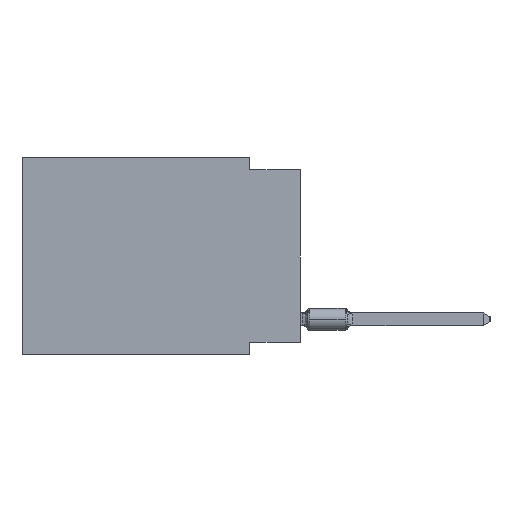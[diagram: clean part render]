
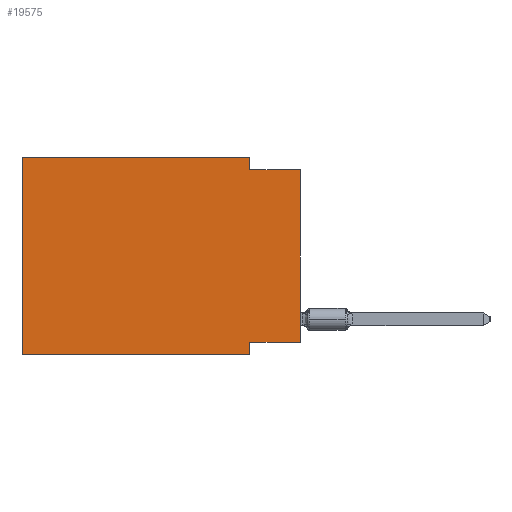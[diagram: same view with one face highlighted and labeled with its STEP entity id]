
A CAD part, left-side view. The second image highlights one B-rep face of the part: STEP entity #19575.
In plain terms, the highlighted planar face has unit normal (-1, 0, 0).
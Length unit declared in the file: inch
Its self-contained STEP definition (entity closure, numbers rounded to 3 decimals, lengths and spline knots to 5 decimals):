
#99 = CARTESIAN_POINT ( 'NONE',  ( 0., 0.1, -0.365 ) ) ;
#309 = EDGE_CURVE ( 'NONE', #10450, #14583, #4186, .T. ) ;
#503 = LINE ( 'NONE', #7809, #4864 ) ;
#529 = DIRECTION ( 'NONE',  ( 1., 0., 0. ) ) ;
#1106 = ORIENTED_EDGE ( 'NONE', *, *, #4842, .T. ) ;
#1479 = CARTESIAN_POINT ( 'NONE',  ( 0., 0.1, -0.025 ) ) ;
#1708 = CARTESIAN_POINT ( 'NONE',  ( 0., 0.55, 0. ) ) ;
#1975 = VERTEX_POINT ( 'NONE', #2293 ) ;
#2190 = AXIS2_PLACEMENT_3D ( 'NONE', #3456, #529, #7834 ) ;
#2293 = CARTESIAN_POINT ( 'NONE',  ( 0., 0.55, 0. ) ) ;
#2427 = EDGE_CURVE ( 'NONE', #8706, #8449, #21002, .T. ) ;
#3456 = CARTESIAN_POINT ( 'NONE',  ( 0., 0.55, 0. ) ) ;
#3761 = VECTOR ( 'NONE', #18174, 39.37008 ) ;
#4017 = CARTESIAN_POINT ( 'NONE',  ( 0., 0., -0.025 ) ) ;
#4186 = LINE ( 'NONE', #17028, #7358 ) ;
#4235 = DIRECTION ( 'NONE',  ( 0., 0., 1. ) ) ;
#4842 = EDGE_CURVE ( 'NONE', #10450, #8449, #13584, .T. ) ;
#4864 = VECTOR ( 'NONE', #4235, 39.37008 ) ;
#5116 = CARTESIAN_POINT ( 'NONE',  ( 0., 0.55, -0.39 ) ) ;
#5328 = ORIENTED_EDGE ( 'NONE', *, *, #7126, .F. ) ;
#5973 = DIRECTION ( 'NONE',  ( 0., 1., 0. ) ) ;
#5985 = ORIENTED_EDGE ( 'NONE', *, *, #309, .F. ) ;
#6417 = ORIENTED_EDGE ( 'NONE', *, *, #2427, .F. ) ;
#7126 = EDGE_CURVE ( 'NONE', #14583, #19615, #7259, .T. ) ;
#7259 = LINE ( 'NONE', #20013, #10514 ) ;
#7358 = VECTOR ( 'NONE', #5973, 39.37008 ) ;
#7434 = DIRECTION ( 'NONE',  ( 0., -1., 0. ) ) ;
#7547 = CARTESIAN_POINT ( 'NONE',  ( 0., 0.55, -0.39 ) ) ;
#7809 = CARTESIAN_POINT ( 'NONE',  ( 0., 0.55, 0. ) ) ;
#7834 = DIRECTION ( 'NONE',  ( 0., 0., -1. ) ) ;
#7867 = VECTOR ( 'NONE', #20658, 39.37008 ) ;
#8103 = LINE ( 'NONE', #7547, #23651 ) ;
#8190 = EDGE_CURVE ( 'NONE', #12442, #19615, #8103, .T. ) ;
#8449 = VERTEX_POINT ( 'NONE', #4017 ) ;
#8706 = VERTEX_POINT ( 'NONE', #1479 ) ;
#8985 = EDGE_CURVE ( 'NONE', #12442, #1975, #503, .T. ) ;
#9356 = VECTOR ( 'NONE', #17526, 39.37008 ) ;
#9798 = CARTESIAN_POINT ( 'NONE',  ( 0., 0., -0.025 ) ) ;
#10450 = VERTEX_POINT ( 'NONE', #13456 ) ;
#10514 = VECTOR ( 'NONE', #16394, 39.37008 ) ;
#11461 = ORIENTED_EDGE ( 'NONE', *, *, #12054, .F. ) ;
#12054 = EDGE_CURVE ( 'NONE', #22132, #8706, #15228, .T. ) ;
#12442 = VERTEX_POINT ( 'NONE', #5116 ) ;
#12765 = ORIENTED_EDGE ( 'NONE', *, *, #8985, .F. ) ;
#13304 = CARTESIAN_POINT ( 'NONE',  ( 0., 0.1, 0. ) ) ;
#13456 = CARTESIAN_POINT ( 'NONE',  ( 0., 0., -0.365 ) ) ;
#13584 = LINE ( 'NONE', #19462, #9356 ) ;
#14069 = LINE ( 'NONE', #1708, #3761 ) ;
#14229 = CARTESIAN_POINT ( 'NONE',  ( 0., 0.1, 0. ) ) ;
#14583 = VERTEX_POINT ( 'NONE', #99 ) ;
#15179 = FACE_OUTER_BOUND ( 'NONE', #19804, .T. ) ;
#15228 = LINE ( 'NONE', #13304, #7867 ) ;
#16394 = DIRECTION ( 'NONE',  ( 0., 0., -1. ) ) ;
#17028 = CARTESIAN_POINT ( 'NONE',  ( 0., 0., -0.365 ) ) ;
#17526 = DIRECTION ( 'NONE',  ( 0., 0., 1. ) ) ;
#18174 = DIRECTION ( 'NONE',  ( 0., -1., 0. ) ) ;
#18807 = CARTESIAN_POINT ( 'NONE',  ( 0., 0.1, -0.39 ) ) ;
#19462 = CARTESIAN_POINT ( 'NONE',  ( 0., 0., 0. ) ) ;
#19575 = ADVANCED_FACE ( 'NONE', ( #15179 ), #23620, .F. ) ;
#19615 = VERTEX_POINT ( 'NONE', #18807 ) ;
#19804 = EDGE_LOOP ( 'NONE', ( #1106, #6417, #11461, #20324, #12765, #20899, #5328, #5985 ) ) ;
#19908 = EDGE_CURVE ( 'NONE', #1975, #22132, #14069, .T. ) ;
#20013 = CARTESIAN_POINT ( 'NONE',  ( 0., 0.1, -0.39 ) ) ;
#20324 = ORIENTED_EDGE ( 'NONE', *, *, #19908, .F. ) ;
#20658 = DIRECTION ( 'NONE',  ( 0., 0., -1. ) ) ;
#20887 = DIRECTION ( 'NONE',  ( 0., -1., 0. ) ) ;
#20899 = ORIENTED_EDGE ( 'NONE', *, *, #8190, .T. ) ;
#21002 = LINE ( 'NONE', #9798, #22410 ) ;
#22132 = VERTEX_POINT ( 'NONE', #14229 ) ;
#22410 = VECTOR ( 'NONE', #20887, 39.37008 ) ;
#23620 = PLANE ( 'NONE',  #2190 ) ;
#23651 = VECTOR ( 'NONE', #7434, 39.37008 ) ;
